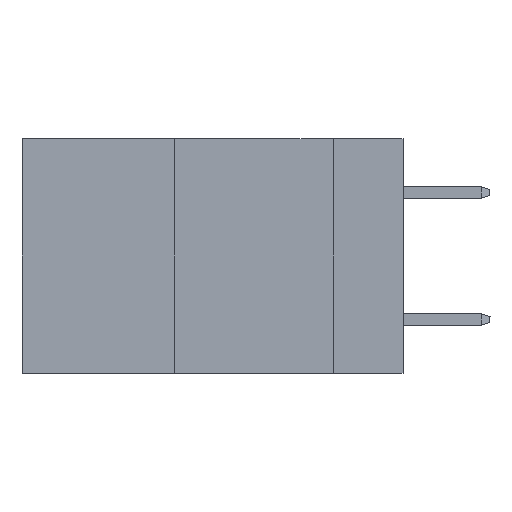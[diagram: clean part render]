
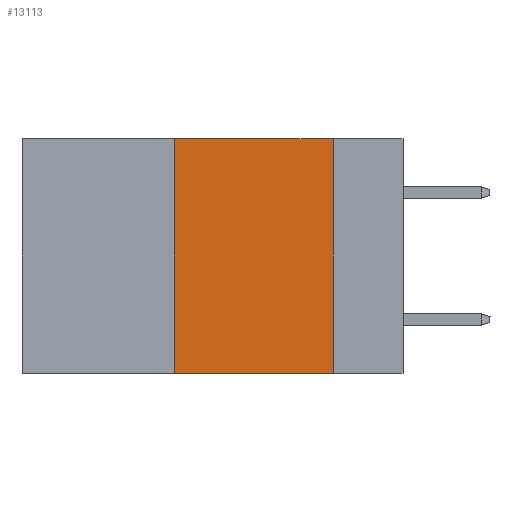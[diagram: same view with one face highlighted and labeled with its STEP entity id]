
A CAD part, left-side view. The second image highlights one B-rep face of the part: STEP entity #13113.
In plain terms, the highlighted planar face has unit normal (-1, 0, 0).
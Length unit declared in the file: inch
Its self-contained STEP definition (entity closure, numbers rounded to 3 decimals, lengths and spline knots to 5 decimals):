
#283 = CARTESIAN_POINT ( 'NONE',  ( 0., 0.6, -0.37 ) ) ;
#1909 = VERTEX_POINT ( 'NONE', #24402 ) ;
#2050 = CARTESIAN_POINT ( 'NONE',  ( 0., 0.6, 0. ) ) ;
#2854 = VECTOR ( 'NONE', #32293, 39.37008 ) ;
#7965 = CARTESIAN_POINT ( 'NONE',  ( 0., 0.36, 0. ) ) ;
#8543 = DIRECTION ( 'NONE',  ( 0., 0., -1. ) ) ;
#8760 = FACE_OUTER_BOUND ( 'NONE', #35886, .T. ) ;
#11629 = DIRECTION ( 'NONE',  ( 0., 0., 1. ) ) ;
#12130 = EDGE_CURVE ( 'NONE', #38521, #22415, #34718, .T. ) ;
#13078 = ORIENTED_EDGE ( 'NONE', *, *, #33894, .F. ) ;
#13095 = DIRECTION ( 'NONE',  ( 0., -1., 0. ) ) ;
#13113 = ADVANCED_FACE ( 'NONE', ( #8760 ), #20607, .F. ) ;
#14464 = CARTESIAN_POINT ( 'NONE',  ( 0., 0.36, 0. ) ) ;
#14961 = CARTESIAN_POINT ( 'NONE',  ( 0., 0.11, -0.37 ) ) ;
#18581 = CARTESIAN_POINT ( 'NONE',  ( 0., 0.6, 0. ) ) ;
#19848 = CARTESIAN_POINT ( 'NONE',  ( 0., 0.11, 0. ) ) ;
#20607 = PLANE ( 'NONE',  #22197 ) ;
#22197 = AXIS2_PLACEMENT_3D ( 'NONE', #2050, #32852, #8543 ) ;
#22415 = VERTEX_POINT ( 'NONE', #14961 ) ;
#22545 = ORIENTED_EDGE ( 'NONE', *, *, #12130, .T. ) ;
#24083 = EDGE_CURVE ( 'NONE', #1909, #22415, #31881, .T. ) ;
#24402 = CARTESIAN_POINT ( 'NONE',  ( 0., 0.11, 0. ) ) ;
#24666 = VECTOR ( 'NONE', #11629, 39.37008 ) ;
#25512 = LINE ( 'NONE', #18581, #26401 ) ;
#25725 = CARTESIAN_POINT ( 'NONE',  ( 0., 0.36, -0.37 ) ) ;
#26401 = VECTOR ( 'NONE', #37132, 39.37008 ) ;
#27948 = ORIENTED_EDGE ( 'NONE', *, *, #40015, .F. ) ;
#31881 = LINE ( 'NONE', #19848, #2854 ) ;
#32293 = DIRECTION ( 'NONE',  ( 0., 0., -1. ) ) ;
#32852 = DIRECTION ( 'NONE',  ( 1., 0., 0. ) ) ;
#33894 = EDGE_CURVE ( 'NONE', #38172, #1909, #25512, .T. ) ;
#34718 = LINE ( 'NONE', #283, #37811 ) ;
#35886 = EDGE_LOOP ( 'NONE', ( #36975, #13078, #27948, #22545 ) ) ;
#36975 = ORIENTED_EDGE ( 'NONE', *, *, #24083, .F. ) ;
#37132 = DIRECTION ( 'NONE',  ( 0., -1., 0. ) ) ;
#37811 = VECTOR ( 'NONE', #13095, 39.37008 ) ;
#38172 = VERTEX_POINT ( 'NONE', #14464 ) ;
#38521 = VERTEX_POINT ( 'NONE', #25725 ) ;
#38748 = LINE ( 'NONE', #7965, #24666 ) ;
#40015 = EDGE_CURVE ( 'NONE', #38521, #38172, #38748, .T. ) ;
